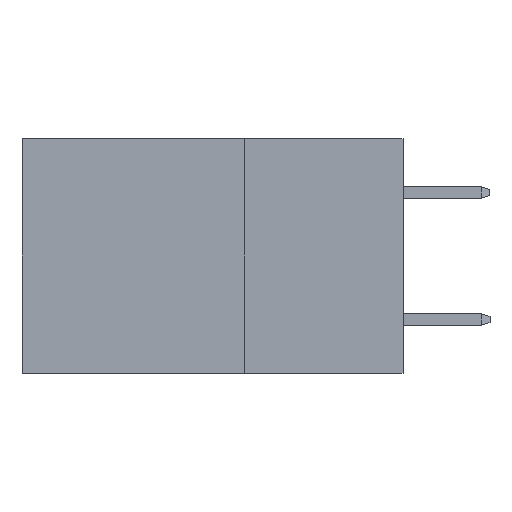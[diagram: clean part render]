
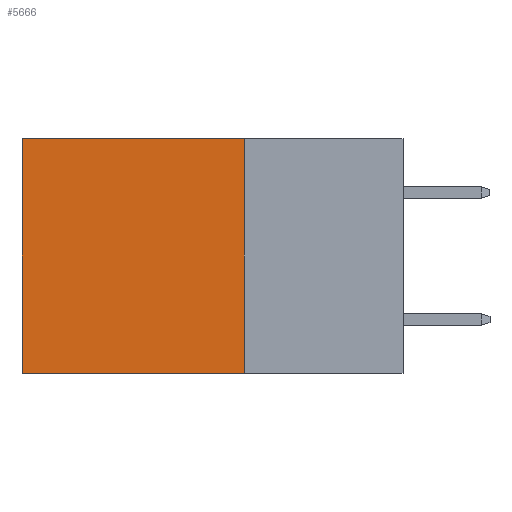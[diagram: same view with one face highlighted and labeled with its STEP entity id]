
A CAD part, left-side view. The second image highlights one B-rep face of the part: STEP entity #5666.
In plain terms, the highlighted planar face has unit normal (-1, 0, 0).
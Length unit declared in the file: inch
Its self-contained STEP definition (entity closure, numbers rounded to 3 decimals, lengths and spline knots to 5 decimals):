
#178 = EDGE_CURVE ( 'NONE', #16030, #7813, #17260, .T. ) ;
#186 = ORIENTED_EDGE ( 'NONE', *, *, #6611, .F. ) ;
#959 = DIRECTION ( 'NONE',  ( 0., 0., -1. ) ) ;
#989 = ORIENTED_EDGE ( 'NONE', *, *, #9740, .F. ) ;
#1274 = VECTOR ( 'NONE', #8204, 39.37008 ) ;
#1619 = CARTESIAN_POINT ( 'NONE',  ( 0.2875, 0.25, 0. ) ) ;
#1670 = CARTESIAN_POINT ( 'NONE',  ( 0.2875, 0.25, 0. ) ) ;
#1737 = AXIS2_PLACEMENT_3D ( 'NONE', #1670, #13935, #959 ) ;
#2126 = VERTEX_POINT ( 'NONE', #5218 ) ;
#2835 = LINE ( 'NONE', #13441, #1274 ) ;
#3679 = VECTOR ( 'NONE', #7656, 39.37008 ) ;
#5218 = CARTESIAN_POINT ( 'NONE',  ( 0.2875, 0.25, -0.37 ) ) ;
#5666 = ADVANCED_FACE ( 'NONE', ( #16318 ), #8349, .F. ) ;
#5726 = CARTESIAN_POINT ( 'NONE',  ( 0.2875, 0.6, 0. ) ) ;
#6538 = CARTESIAN_POINT ( 'NONE',  ( 0.2875, 0.6, 0. ) ) ;
#6611 = EDGE_CURVE ( 'NONE', #2126, #7813, #15443, .T. ) ;
#6715 = DIRECTION ( 'NONE',  ( 0., 0., -1. ) ) ;
#7656 = DIRECTION ( 'NONE',  ( 0., 1., 0. ) ) ;
#7813 = VERTEX_POINT ( 'NONE', #12233 ) ;
#8067 = VECTOR ( 'NONE', #6715, 39.37008 ) ;
#8204 = DIRECTION ( 'NONE',  ( 0., 1., 0. ) ) ;
#8349 = PLANE ( 'NONE',  #1737 ) ;
#8623 = LINE ( 'NONE', #1619, #16958 ) ;
#9050 = ORIENTED_EDGE ( 'NONE', *, *, #9536, .T. ) ;
#9329 = CARTESIAN_POINT ( 'NONE',  ( 0.2875, 0.25, 0. ) ) ;
#9536 = EDGE_CURVE ( 'NONE', #16425, #16030, #2835, .T. ) ;
#9740 = EDGE_CURVE ( 'NONE', #16425, #2126, #8623, .T. ) ;
#12233 = CARTESIAN_POINT ( 'NONE',  ( 0.2875, 0.6, -0.37 ) ) ;
#12425 = EDGE_LOOP ( 'NONE', ( #16664, #186, #989, #9050 ) ) ;
#13441 = CARTESIAN_POINT ( 'NONE',  ( 0.2875, 0.25, 0. ) ) ;
#13935 = DIRECTION ( 'NONE',  ( 1., 0., 0. ) ) ;
#14127 = CARTESIAN_POINT ( 'NONE',  ( 0.2875, 0.25, -0.37 ) ) ;
#15190 = DIRECTION ( 'NONE',  ( 0., 0., -1. ) ) ;
#15443 = LINE ( 'NONE', #14127, #3679 ) ;
#16030 = VERTEX_POINT ( 'NONE', #5726 ) ;
#16318 = FACE_OUTER_BOUND ( 'NONE', #12425, .T. ) ;
#16425 = VERTEX_POINT ( 'NONE', #9329 ) ;
#16664 = ORIENTED_EDGE ( 'NONE', *, *, #178, .T. ) ;
#16958 = VECTOR ( 'NONE', #15190, 39.37008 ) ;
#17260 = LINE ( 'NONE', #6538, #8067 ) ;
